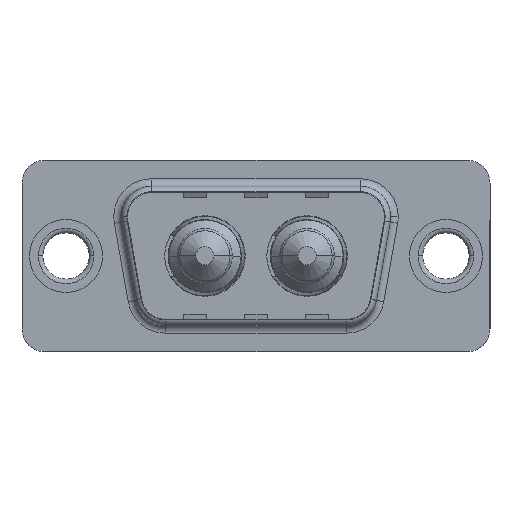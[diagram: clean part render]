
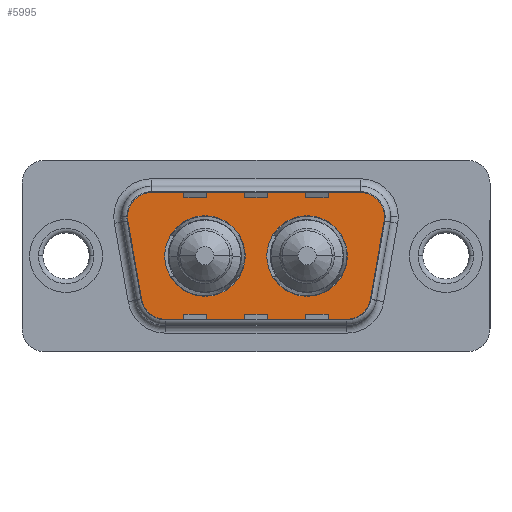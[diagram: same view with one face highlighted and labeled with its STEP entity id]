
A CAD part, top view. The second image highlights one B-rep face of the part: STEP entity #5995.
In plain terms, the highlighted planar face has unit normal (0, 0, 1).
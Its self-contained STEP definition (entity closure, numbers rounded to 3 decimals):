
#105 = CARTESIAN_POINT ( 'NONE',  ( 18.51, 0., 0. ) ) ;
#237 = EDGE_CURVE ( 'NONE', #473, #1687, #4108, .T. ) ;
#249 = EDGE_CURVE ( 'NONE', #4432, #1078, #3408, .T. ) ;
#252 = AXIS2_PLACEMENT_3D ( 'NONE', #2594, #7936, #3347 ) ;
#322 = EDGE_CURVE ( 'NONE', #1078, #1667, #9039, .T. ) ;
#421 = ORIENTED_EDGE ( 'NONE', *, *, #237, .T. ) ;
#441 = FACE_BOUND ( 'NONE', #6444, .T. ) ;
#446 = DIRECTION ( 'NONE',  ( 0., 0., 1. ) ) ;
#473 = VERTEX_POINT ( 'NONE', #2896 ) ;
#474 = ORIENTED_EDGE ( 'NONE', *, *, #9749, .T. ) ;
#524 = CARTESIAN_POINT ( 'NONE',  ( 9.14, 0., 0. ) ) ;
#707 = ORIENTED_EDGE ( 'NONE', *, *, #7689, .T. ) ;
#714 = DIRECTION ( 'NONE',  ( -1., 0., 0. ) ) ;
#784 = CARTESIAN_POINT ( 'NONE',  ( 6.459, -4.9, 0. ) ) ;
#859 = CARTESIAN_POINT ( 'NONE',  ( 18.541, -2.9, 0. ) ) ;
#944 = ORIENTED_EDGE ( 'NONE', *, *, #4816, .T. ) ;
#998 = CARTESIAN_POINT ( 'NONE',  ( 21.564, 2.9, 0. ) ) ;
#1023 = CARTESIAN_POINT ( 'NONE',  ( 18.541, -4.9, 0. ) ) ;
#1078 = VERTEX_POINT ( 'NONE', #3079 ) ;
#1142 = CIRCLE ( 'NONE', #7918, 2.65 ) ;
#1263 = VECTOR ( 'NONE', #8688, 1000. ) ;
#1405 = VECTOR ( 'NONE', #5598, 1000. ) ;
#1571 = CIRCLE ( 'NONE', #3805, 2. ) ;
#1667 = VERTEX_POINT ( 'NONE', #3957 ) ;
#1671 = ORIENTED_EDGE ( 'NONE', *, *, #8552, .F. ) ;
#1687 = VERTEX_POINT ( 'NONE', #7020 ) ;
#1883 = VECTOR ( 'NONE', #7584, 1000. ) ;
#1885 = CARTESIAN_POINT ( 'NONE',  ( 9.14, 0., 0. ) ) ;
#1968 = CIRCLE ( 'NONE', #8349, 2. ) ;
#2016 = VERTEX_POINT ( 'NONE', #6397 ) ;
#2209 = VERTEX_POINT ( 'NONE', #9137 ) ;
#2342 = DIRECTION ( 'NONE',  ( 1., 0., 0. ) ) ;
#2349 = AXIS2_PLACEMENT_3D ( 'NONE', #859, #446, #7004 ) ;
#2407 = DIRECTION ( 'NONE',  ( 1., 0., 0. ) ) ;
#2454 = EDGE_CURVE ( 'NONE', #7888, #4432, #3716, .T. ) ;
#2464 = FACE_BOUND ( 'NONE', #3764, .T. ) ;
#2477 = VERTEX_POINT ( 'NONE', #105 ) ;
#2594 = CARTESIAN_POINT ( 'NONE',  ( 15.86, 0., 0. ) ) ;
#2603 = VERTEX_POINT ( 'NONE', #1023 ) ;
#2637 = DIRECTION ( 'NONE',  ( 1., 0., 0. ) ) ;
#2775 = DIRECTION ( 'NONE',  ( 0., 0., 1. ) ) ;
#2777 = CIRCLE ( 'NONE', #5073, 2. ) ;
#2879 = CARTESIAN_POINT ( 'NONE',  ( 6.49, 0., 0. ) ) ;
#2896 = CARTESIAN_POINT ( 'NONE',  ( 20.511, -3.247, 0. ) ) ;
#2950 = CARTESIAN_POINT ( 'NONE',  ( 5.436, 2.9, 0. ) ) ;
#3035 = AXIS2_PLACEMENT_3D ( 'NONE', #524, #5392, #2342 ) ;
#3079 = CARTESIAN_POINT ( 'NONE',  ( 5.436, 4.9, 0. ) ) ;
#3226 = ORIENTED_EDGE ( 'NONE', *, *, #7305, .F. ) ;
#3342 = CIRCLE ( 'NONE', #3035, 2.65 ) ;
#3347 = DIRECTION ( 'NONE',  ( 1., 0., 0. ) ) ;
#3366 = DIRECTION ( 'NONE',  ( 0., 0., 1. ) ) ;
#3408 = LINE ( 'NONE', #4542, #1405 ) ;
#3620 = CIRCLE ( 'NONE', #9577, 2.65 ) ;
#3665 = VERTEX_POINT ( 'NONE', #2879 ) ;
#3687 = EDGE_CURVE ( 'NONE', #3665, #2209, #3342, .T. ) ;
#3716 = CIRCLE ( 'NONE', #9283, 2. ) ;
#3764 = EDGE_LOOP ( 'NONE', ( #1671, #4719 ) ) ;
#3805 = AXIS2_PLACEMENT_3D ( 'NONE', #9271, #3366, #5969 ) ;
#3845 = CARTESIAN_POINT ( 'NONE',  ( 18.541, -2.9, 0. ) ) ;
#3957 = CARTESIAN_POINT ( 'NONE',  ( 3.466, 2.553, 0. ) ) ;
#4078 = CARTESIAN_POINT ( 'NONE',  ( 6.459, -4.9, 0. ) ) ;
#4108 = LINE ( 'NONE', #9190, #1883 ) ;
#4432 = VERTEX_POINT ( 'NONE', #7783 ) ;
#4466 = CARTESIAN_POINT ( 'NONE',  ( 19.564, 2.9, 0. ) ) ;
#4542 = CARTESIAN_POINT ( 'NONE',  ( 5.436, 4.9, 0. ) ) ;
#4549 = LINE ( 'NONE', #6159, #6332 ) ;
#4609 = DIRECTION ( 'NONE',  ( 1., 0., 0. ) ) ;
#4626 = AXIS2_PLACEMENT_3D ( 'NONE', #2950, #5639, #2407 ) ;
#4719 = ORIENTED_EDGE ( 'NONE', *, *, #8724, .F. ) ;
#4816 = EDGE_CURVE ( 'NONE', #2016, #6199, #1571, .T. ) ;
#5073 = AXIS2_PLACEMENT_3D ( 'NONE', #3845, #9211, #4609 ) ;
#5247 = DIRECTION ( 'NONE',  ( -1., 0., 0. ) ) ;
#5362 = ORIENTED_EDGE ( 'NONE', *, *, #249, .T. ) ;
#5392 = DIRECTION ( 'NONE',  ( 0., 0., 1. ) ) ;
#5598 = DIRECTION ( 'NONE',  ( -1., 0., 0. ) ) ;
#5639 = DIRECTION ( 'NONE',  ( 0., 0., 1. ) ) ;
#5969 = DIRECTION ( 'NONE',  ( -1., 0., 0. ) ) ;
#5995 = ADVANCED_FACE ( 'NONE', ( #2464, #441, #8799 ), #9304, .T. ) ;
#6159 = CARTESIAN_POINT ( 'NONE',  ( 3.466, 2.553, 0. ) ) ;
#6199 = VERTEX_POINT ( 'NONE', #784 ) ;
#6332 = VECTOR ( 'NONE', #8504, 1000. ) ;
#6343 = CIRCLE ( 'NONE', #252, 2.65 ) ;
#6397 = CARTESIAN_POINT ( 'NONE',  ( 4.489, -3.247, 0. ) ) ;
#6444 = EDGE_LOOP ( 'NONE', ( #3226, #9533 ) ) ;
#6563 = ORIENTED_EDGE ( 'NONE', *, *, #2454, .T. ) ;
#6792 = ORIENTED_EDGE ( 'NONE', *, *, #322, .T. ) ;
#7004 = DIRECTION ( 'NONE',  ( 1., 0., 0. ) ) ;
#7013 = VERTEX_POINT ( 'NONE', #8317 ) ;
#7020 = CARTESIAN_POINT ( 'NONE',  ( 21.534, 2.553, 0. ) ) ;
#7181 = DIRECTION ( 'NONE',  ( 0., 0., 1. ) ) ;
#7305 = EDGE_CURVE ( 'NONE', #2209, #3665, #3620, .T. ) ;
#7345 = CARTESIAN_POINT ( 'NONE',  ( 15.86, 0., 0. ) ) ;
#7563 = EDGE_CURVE ( 'NONE', #1687, #7888, #1968, .T. ) ;
#7584 = DIRECTION ( 'NONE',  ( 0.174, 0.985, 0. ) ) ;
#7689 = EDGE_CURVE ( 'NONE', #2603, #473, #2777, .T. ) ;
#7783 = CARTESIAN_POINT ( 'NONE',  ( 19.564, 4.9, 0. ) ) ;
#7811 = LINE ( 'NONE', #4078, #1263 ) ;
#7888 = VERTEX_POINT ( 'NONE', #998 ) ;
#7918 = AXIS2_PLACEMENT_3D ( 'NONE', #7345, #2775, #8130 ) ;
#7936 = DIRECTION ( 'NONE',  ( 0., 0., 1. ) ) ;
#8130 = DIRECTION ( 'NONE',  ( 1., 0., 0. ) ) ;
#8317 = CARTESIAN_POINT ( 'NONE',  ( 13.21, 0., 0. ) ) ;
#8349 = AXIS2_PLACEMENT_3D ( 'NONE', #4466, #9836, #5247 ) ;
#8504 = DIRECTION ( 'NONE',  ( 0.174, -0.985, 0. ) ) ;
#8552 = EDGE_CURVE ( 'NONE', #2477, #7013, #6343, .T. ) ;
#8616 = ORIENTED_EDGE ( 'NONE', *, *, #7563, .T. ) ;
#8688 = DIRECTION ( 'NONE',  ( 1., 0., 0. ) ) ;
#8724 = EDGE_CURVE ( 'NONE', #7013, #2477, #1142, .T. ) ;
#8781 = EDGE_LOOP ( 'NONE', ( #707, #421, #8616, #6563, #5362, #6792, #9632, #944, #474 ) ) ;
#8799 = FACE_OUTER_BOUND ( 'NONE', #8781, .T. ) ;
#9039 = CIRCLE ( 'NONE', #4626, 2. ) ;
#9080 = EDGE_CURVE ( 'NONE', #1667, #2016, #4549, .T. ) ;
#9137 = CARTESIAN_POINT ( 'NONE',  ( 11.79, 0., 0. ) ) ;
#9190 = CARTESIAN_POINT ( 'NONE',  ( 21.534, 2.553, 0. ) ) ;
#9211 = DIRECTION ( 'NONE',  ( 0., 0., 1. ) ) ;
#9271 = CARTESIAN_POINT ( 'NONE',  ( 6.459, -2.9, 0. ) ) ;
#9283 = AXIS2_PLACEMENT_3D ( 'NONE', #9428, #9455, #714 ) ;
#9304 = PLANE ( 'NONE',  #2349 ) ;
#9428 = CARTESIAN_POINT ( 'NONE',  ( 19.564, 2.9, 0. ) ) ;
#9455 = DIRECTION ( 'NONE',  ( 0., 0., 1. ) ) ;
#9533 = ORIENTED_EDGE ( 'NONE', *, *, #3687, .F. ) ;
#9577 = AXIS2_PLACEMENT_3D ( 'NONE', #1885, #7181, #2637 ) ;
#9632 = ORIENTED_EDGE ( 'NONE', *, *, #9080, .T. ) ;
#9749 = EDGE_CURVE ( 'NONE', #6199, #2603, #7811, .T. ) ;
#9836 = DIRECTION ( 'NONE',  ( 0., 0., 1. ) ) ;
